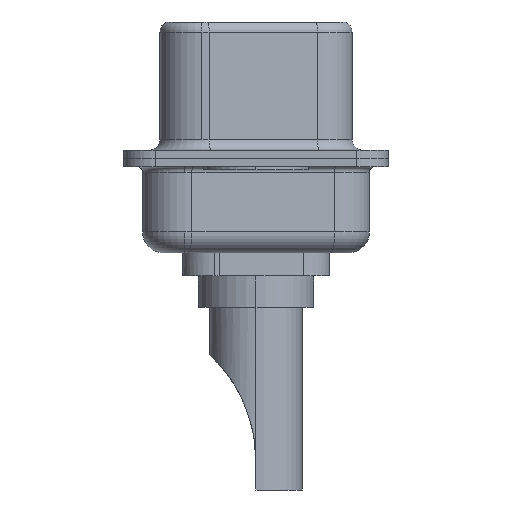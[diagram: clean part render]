
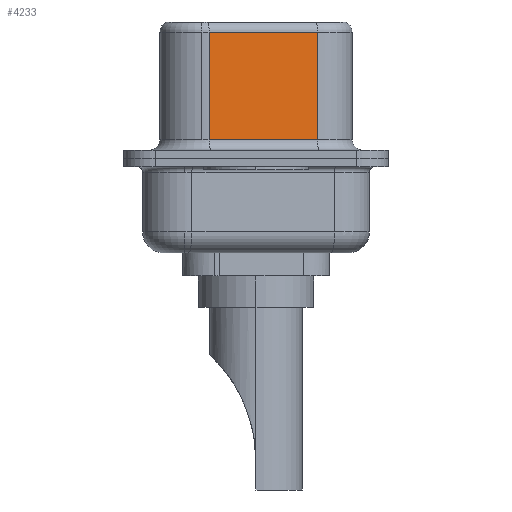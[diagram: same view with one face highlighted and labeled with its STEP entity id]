
A CAD part, left-side view. The second image highlights one B-rep face of the part: STEP entity #4233.
In plain terms, the highlighted planar face has unit normal (-0.985, -0.174, 0).
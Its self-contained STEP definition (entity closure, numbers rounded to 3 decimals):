
#21 = LINE ( 'NONE', #1114, #14054 ) ;
#92 = DIRECTION ( 'NONE',  ( 0., 0., -1. ) ) ;
#184 = CARTESIAN_POINT ( 'NONE',  ( 4.565, -2.927, 6.02 ) ) ;
#586 = VERTEX_POINT ( 'NONE', #8262 ) ;
#756 = DIRECTION ( 'NONE',  ( 0., 0., -1. ) ) ;
#1114 = CARTESIAN_POINT ( 'NONE',  ( 4.565, -2.927, 0.9 ) ) ;
#1158 = LINE ( 'NONE', #8599, #12384 ) ;
#2193 = VERTEX_POINT ( 'NONE', #9502 ) ;
#2537 = VECTOR ( 'NONE', #92, 1000. ) ;
#2635 = VERTEX_POINT ( 'NONE', #184 ) ;
#2923 = CARTESIAN_POINT ( 'NONE',  ( 3.655, 2.233, 6.02 ) ) ;
#3405 = CARTESIAN_POINT ( 'NONE',  ( 4.565, -2.927, 6.52 ) ) ;
#3504 = CARTESIAN_POINT ( 'NONE',  ( 4.565, -2.927, 6.52 ) ) ;
#4233 = ADVANCED_FACE ( 'NONE', ( #12386 ), #13949, .F. ) ;
#5082 = CARTESIAN_POINT ( 'NONE',  ( 3.655, 2.233, 6.52 ) ) ;
#5378 = LINE ( 'NONE', #3405, #2537 ) ;
#5768 = ORIENTED_EDGE ( 'NONE', *, *, #12058, .T. ) ;
#6472 = ORIENTED_EDGE ( 'NONE', *, *, #9787, .T. ) ;
#7792 = AXIS2_PLACEMENT_3D ( 'NONE', #3504, #8017, #9436 ) ;
#7820 = VERTEX_POINT ( 'NONE', #2923 ) ;
#8017 = DIRECTION ( 'NONE',  ( 0.985, 0.174, 0. ) ) ;
#8262 = CARTESIAN_POINT ( 'NONE',  ( 4.565, -2.927, 0.9 ) ) ;
#8584 = DIRECTION ( 'NONE',  ( -0.174, 0.985, 0. ) ) ;
#8599 = CARTESIAN_POINT ( 'NONE',  ( 4.565, -2.927, 6.02 ) ) ;
#9436 = DIRECTION ( 'NONE',  ( -0.174, 0.985, 0. ) ) ;
#9502 = CARTESIAN_POINT ( 'NONE',  ( 3.655, 2.233, 0.9 ) ) ;
#9787 = EDGE_CURVE ( 'NONE', #2635, #7820, #1158, .T. ) ;
#9894 = DIRECTION ( 'NONE',  ( 0.174, -0.985, 0. ) ) ;
#10659 = EDGE_CURVE ( 'NONE', #2635, #586, #5378, .T. ) ;
#10882 = EDGE_LOOP ( 'NONE', ( #12856, #6472, #13861, #5768 ) ) ;
#11862 = EDGE_CURVE ( 'NONE', #7820, #2193, #13690, .T. ) ;
#12058 = EDGE_CURVE ( 'NONE', #2193, #586, #21, .T. ) ;
#12384 = VECTOR ( 'NONE', #8584, 1000. ) ;
#12386 = FACE_OUTER_BOUND ( 'NONE', #10882, .T. ) ;
#12856 = ORIENTED_EDGE ( 'NONE', *, *, #10659, .F. ) ;
#13362 = VECTOR ( 'NONE', #756, 1000. ) ;
#13690 = LINE ( 'NONE', #5082, #13362 ) ;
#13861 = ORIENTED_EDGE ( 'NONE', *, *, #11862, .T. ) ;
#13949 = PLANE ( 'NONE',  #7792 ) ;
#14054 = VECTOR ( 'NONE', #9894, 1000. ) ;
